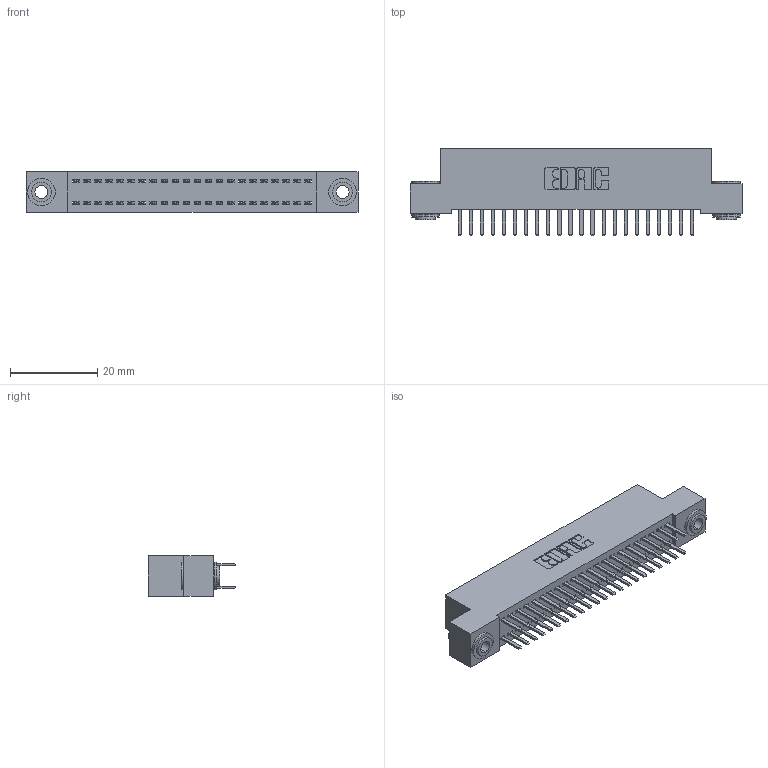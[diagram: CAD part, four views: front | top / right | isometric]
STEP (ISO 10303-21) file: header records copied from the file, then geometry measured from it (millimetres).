
FILE_DESCRIPTION (( 'STEP AP203' ), '1' );
FILE_NAME ('342-044-520-203.STEP', '2018-08-12T14:15:22', ( '' ), ( '' ), 'SwSTEP 2.0', 'SolidWorks 2016', '' );
FILE_SCHEMA (( 'CONFIG_CONTROL_DESIGN' ));
Length unit declared in the file: inch
Products named in the file (4): 342 Part_.156 TH; 345-292-001_345-293-120; 342-250-002_345-250-002-102; 342-044-520-203
Assembly tree (47 placements, depth 2):
  342-044-520-203
    342 Part_.156 TH
    345-292-001_345-293-120  x44
    342-250-002_345-250-002-102  x2
Bounding box: 76.2 x 20.02 x 9.4 mm (x, y, z)
Volume: 6755.4 mm3; surface area: 10671.7 mm2
Topology: 47 solids, 47 shells, 2612 faces, 7547 edges, 4910 vertices
Faces by surface type: plane 1748, cylinder 856, cone 8
Entity records: 17372 total; most frequent: CARTESIAN_POINT 2889, ORIENTED_EDGE 2806, DIRECTION 2525, EDGE_CURVE 1403, VECTOR 1247, LINE 1247, VERTEX_POINT 930, AXIS2_PLACEMENT_3D 639
